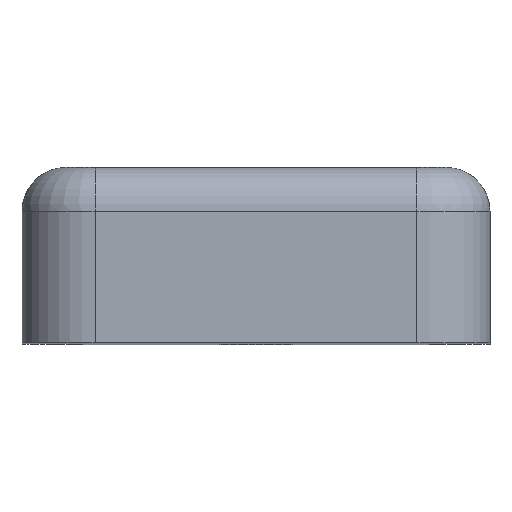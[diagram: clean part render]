
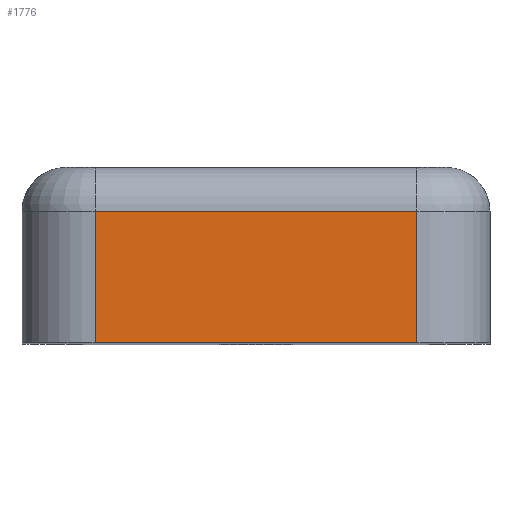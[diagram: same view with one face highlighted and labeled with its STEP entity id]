
A CAD part, top view. The second image highlights one B-rep face of the part: STEP entity #1776.
In plain terms, the highlighted planar face has unit normal (0, 0, 1).
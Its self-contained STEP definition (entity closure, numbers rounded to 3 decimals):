
#105 = AXIS2_PLACEMENT_3D ( 'NONE', #1095, #1256, #296 ) ;
#147 = LINE ( 'NONE', #1264, #1389 ) ;
#292 = VERTEX_POINT ( 'NONE', #1077 ) ;
#296 = DIRECTION ( 'NONE',  ( -1., 0., 0. ) ) ;
#347 = CARTESIAN_POINT ( 'NONE',  ( 11., 0., 35.5 ) ) ;
#382 = EDGE_CURVE ( 'NONE', #755, #1189, #559, .T. ) ;
#480 = CARTESIAN_POINT ( 'NONE',  ( -16., 0., 35.5 ) ) ;
#481 = VECTOR ( 'NONE', #1284, 1000. ) ;
#518 = VECTOR ( 'NONE', #1160, 1000. ) ;
#559 = LINE ( 'NONE', #1344, #518 ) ;
#703 = EDGE_CURVE ( 'NONE', #1189, #1933, #975, .T. ) ;
#755 = VERTEX_POINT ( 'NONE', #1424 ) ;
#783 = PLANE ( 'NONE',  #105 ) ;
#811 = DIRECTION ( 'NONE',  ( 0., 1., 0. ) ) ;
#841 = ORIENTED_EDGE ( 'NONE', *, *, #1019, .T. ) ;
#941 = CARTESIAN_POINT ( 'NONE',  ( -11., 9., 35.5 ) ) ;
#975 = LINE ( 'NONE', #480, #1560 ) ;
#1019 = EDGE_CURVE ( 'NONE', #1933, #292, #147, .T. ) ;
#1032 = EDGE_CURVE ( 'NONE', #292, #755, #1429, .T. ) ;
#1077 = CARTESIAN_POINT ( 'NONE',  ( 11., 9., 35.5 ) ) ;
#1095 = CARTESIAN_POINT ( 'NONE',  ( -16., 2., 35.5 ) ) ;
#1160 = DIRECTION ( 'NONE',  ( 0., -1., 0. ) ) ;
#1189 = VERTEX_POINT ( 'NONE', #1806 ) ;
#1256 = DIRECTION ( 'NONE',  ( 0., 0., -1. ) ) ;
#1264 = CARTESIAN_POINT ( 'NONE',  ( 11., 2., 35.5 ) ) ;
#1284 = DIRECTION ( 'NONE',  ( -1., 0., 0. ) ) ;
#1344 = CARTESIAN_POINT ( 'NONE',  ( -11., 2., 35.5 ) ) ;
#1389 = VECTOR ( 'NONE', #811, 1000. ) ;
#1411 = ORIENTED_EDGE ( 'NONE', *, *, #1032, .T. ) ;
#1424 = CARTESIAN_POINT ( 'NONE',  ( -11., 9., 35.5 ) ) ;
#1429 = LINE ( 'NONE', #941, #481 ) ;
#1431 = DIRECTION ( 'NONE',  ( 1., 0., 0. ) ) ;
#1517 = EDGE_LOOP ( 'NONE', ( #841, #1411, #1887, #1707 ) ) ;
#1560 = VECTOR ( 'NONE', #1431, 1000. ) ;
#1707 = ORIENTED_EDGE ( 'NONE', *, *, #703, .T. ) ;
#1776 = ADVANCED_FACE ( 'NONE', ( #1900 ), #783, .F. ) ;
#1806 = CARTESIAN_POINT ( 'NONE',  ( -11., 0., 35.5 ) ) ;
#1887 = ORIENTED_EDGE ( 'NONE', *, *, #382, .T. ) ;
#1900 = FACE_OUTER_BOUND ( 'NONE', #1517, .T. ) ;
#1933 = VERTEX_POINT ( 'NONE', #347 ) ;
